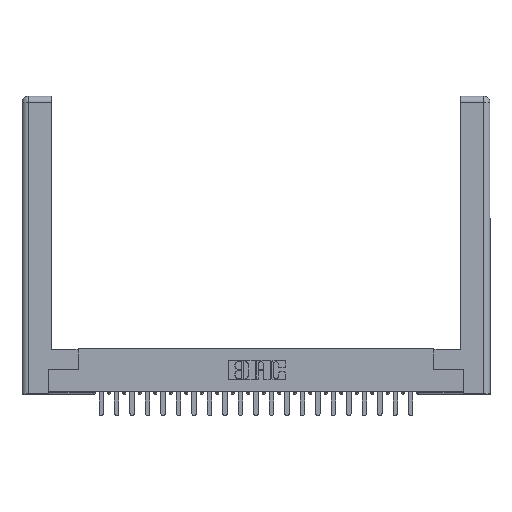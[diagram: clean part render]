
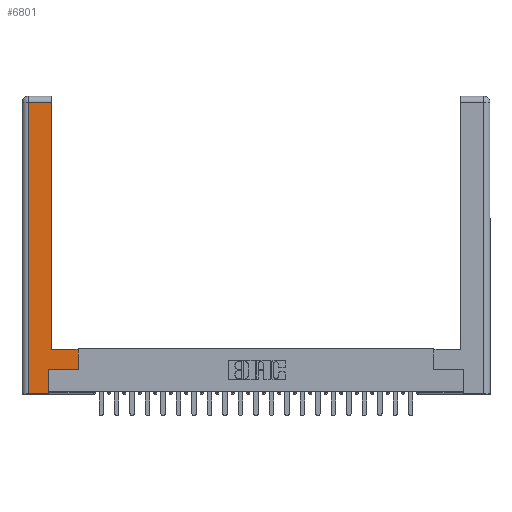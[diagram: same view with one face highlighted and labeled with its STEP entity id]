
A CAD part, top view. The second image highlights one B-rep face of the part: STEP entity #6801.
In plain terms, the highlighted planar face has unit normal (0, 0, 1).
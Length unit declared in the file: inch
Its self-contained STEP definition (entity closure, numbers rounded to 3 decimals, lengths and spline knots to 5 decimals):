
#126 = CARTESIAN_POINT ( 'NONE',  ( 0.265, 0., 0. ) ) ;
#286 = DIRECTION ( 'NONE',  ( 0., 1., 0. ) ) ;
#1006 = EDGE_LOOP ( 'NONE', ( #24029, #22120, #2548, #5242, #1332, #17545, #27796, #20118 ) ) ;
#1332 = ORIENTED_EDGE ( 'NONE', *, *, #8162, .T. ) ;
#1506 = VERTEX_POINT ( 'NONE', #7199 ) ;
#1681 = DIRECTION ( 'NONE',  ( 0., 1., 0. ) ) ;
#2475 = VECTOR ( 'NONE', #22345, 39.37008 ) ;
#2548 = ORIENTED_EDGE ( 'NONE', *, *, #22254, .T. ) ;
#2966 = CARTESIAN_POINT ( 'NONE',  ( 0.565, 0.45, 0. ) ) ;
#4420 = LINE ( 'NONE', #17775, #18888 ) ;
#4995 = VECTOR ( 'NONE', #286, 39.37008 ) ;
#5242 = ORIENTED_EDGE ( 'NONE', *, *, #9186, .T. ) ;
#6518 = LINE ( 'NONE', #14377, #7189 ) ;
#6757 = VERTEX_POINT ( 'NONE', #11842 ) ;
#6801 = ADVANCED_FACE ( 'NONE', ( #22307 ), #12325, .F. ) ;
#7189 = VECTOR ( 'NONE', #16218, 39.37008 ) ;
#7199 = CARTESIAN_POINT ( 'NONE',  ( 0.0615, 2.94, 0. ) ) ;
#7558 = LINE ( 'NONE', #23171, #10895 ) ;
#8162 = EDGE_CURVE ( 'NONE', #11362, #27825, #12704, .T. ) ;
#8169 = LINE ( 'NONE', #11769, #2475 ) ;
#8285 = VECTOR ( 'NONE', #19639, 39.37008 ) ;
#8341 = LINE ( 'NONE', #14759, #22811 ) ;
#8678 = CARTESIAN_POINT ( 'NONE',  ( 0.0615, 0., 0. ) ) ;
#8781 = CARTESIAN_POINT ( 'NONE',  ( 0.295, 3., 0. ) ) ;
#9186 = EDGE_CURVE ( 'NONE', #12331, #11362, #19737, .T. ) ;
#9215 = CARTESIAN_POINT ( 'NONE',  ( 0.295, 0.45, 0. ) ) ;
#9268 = CARTESIAN_POINT ( 'NONE',  ( 0.265, 0.245, 0. ) ) ;
#10895 = VECTOR ( 'NONE', #16539, 39.37008 ) ;
#11263 = VERTEX_POINT ( 'NONE', #2966 ) ;
#11362 = VERTEX_POINT ( 'NONE', #24754 ) ;
#11769 = CARTESIAN_POINT ( 'NONE',  ( 0.295, 0.45, 0. ) ) ;
#11842 = CARTESIAN_POINT ( 'NONE',  ( 0.295, 2.94, 0. ) ) ;
#12325 = PLANE ( 'NONE',  #20753 ) ;
#12331 = VERTEX_POINT ( 'NONE', #8678 ) ;
#12523 = EDGE_CURVE ( 'NONE', #6757, #1506, #4420, .T. ) ;
#12594 = DIRECTION ( 'NONE',  ( -1., 0., 0. ) ) ;
#12704 = LINE ( 'NONE', #15835, #21475 ) ;
#13481 = VERTEX_POINT ( 'NONE', #24114 ) ;
#13560 = DIRECTION ( 'NONE',  ( -1., 0., 0. ) ) ;
#13948 = EDGE_CURVE ( 'NONE', #11263, #20062, #8169, .T. ) ;
#14377 = CARTESIAN_POINT ( 'NONE',  ( 0.0615, 0., 0. ) ) ;
#14679 = CARTESIAN_POINT ( 'NONE',  ( 0., 0., 0. ) ) ;
#14759 = CARTESIAN_POINT ( 'NONE',  ( 0.565, 0.45, 0. ) ) ;
#15835 = CARTESIAN_POINT ( 'NONE',  ( 0.265, 0.245, 0. ) ) ;
#16218 = DIRECTION ( 'NONE',  ( 0., -1., 0. ) ) ;
#16362 = LINE ( 'NONE', #8781, #4995 ) ;
#16539 = DIRECTION ( 'NONE',  ( 1., 0., 0. ) ) ;
#16659 = DIRECTION ( 'NONE',  ( 0., 1., 0. ) ) ;
#17545 = ORIENTED_EDGE ( 'NONE', *, *, #21687, .T. ) ;
#17775 = CARTESIAN_POINT ( 'NONE',  ( 0.0615, 2.94, 0. ) ) ;
#18888 = VECTOR ( 'NONE', #13560, 39.37008 ) ;
#18926 = DIRECTION ( 'NONE',  ( 0., 0., -1. ) ) ;
#19639 = DIRECTION ( 'NONE',  ( 1., 0., 0. ) ) ;
#19737 = LINE ( 'NONE', #126, #8285 ) ;
#20062 = VERTEX_POINT ( 'NONE', #9215 ) ;
#20118 = ORIENTED_EDGE ( 'NONE', *, *, #13948, .T. ) ;
#20357 = EDGE_CURVE ( 'NONE', #20062, #6757, #16362, .T. ) ;
#20753 = AXIS2_PLACEMENT_3D ( 'NONE', #14679, #18926, #12594 ) ;
#21475 = VECTOR ( 'NONE', #16659, 39.37008 ) ;
#21687 = EDGE_CURVE ( 'NONE', #27825, #13481, #7558, .T. ) ;
#22120 = ORIENTED_EDGE ( 'NONE', *, *, #12523, .T. ) ;
#22254 = EDGE_CURVE ( 'NONE', #1506, #12331, #6518, .T. ) ;
#22307 = FACE_OUTER_BOUND ( 'NONE', #1006, .T. ) ;
#22345 = DIRECTION ( 'NONE',  ( -1., 0., 0. ) ) ;
#22811 = VECTOR ( 'NONE', #1681, 39.37008 ) ;
#23171 = CARTESIAN_POINT ( 'NONE',  ( 0.565, 0.245, 0. ) ) ;
#24029 = ORIENTED_EDGE ( 'NONE', *, *, #20357, .T. ) ;
#24114 = CARTESIAN_POINT ( 'NONE',  ( 0.565, 0.245, 0. ) ) ;
#24754 = CARTESIAN_POINT ( 'NONE',  ( 0.265, 0., 0. ) ) ;
#26145 = EDGE_CURVE ( 'NONE', #13481, #11263, #8341, .T. ) ;
#27796 = ORIENTED_EDGE ( 'NONE', *, *, #26145, .T. ) ;
#27825 = VERTEX_POINT ( 'NONE', #9268 ) ;
